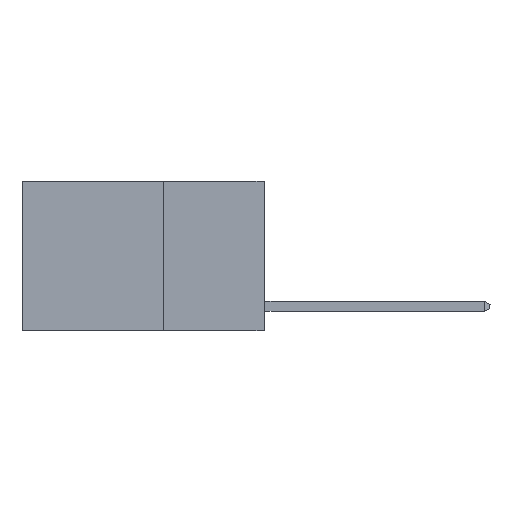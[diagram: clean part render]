
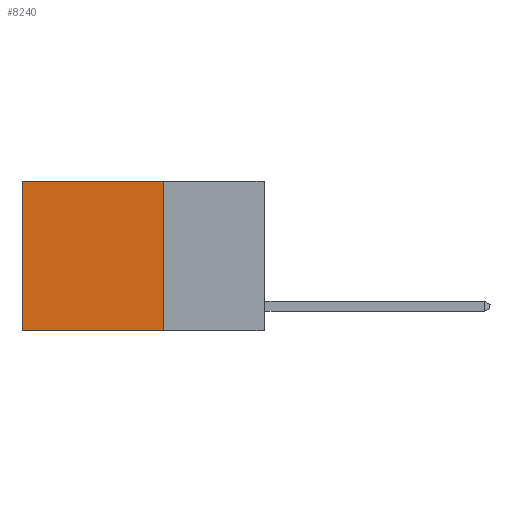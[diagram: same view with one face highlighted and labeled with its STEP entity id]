
A CAD part, left-side view. The second image highlights one B-rep face of the part: STEP entity #8240.
In plain terms, the highlighted planar face has unit normal (-1, 0, 0).
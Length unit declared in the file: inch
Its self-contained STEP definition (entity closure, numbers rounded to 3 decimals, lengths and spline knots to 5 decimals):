
#492 = EDGE_CURVE ( 'NONE', #12961, #1745, #1824, .T. ) ;
#1249 = CARTESIAN_POINT ( 'NONE',  ( 0.2625, 0.6, 0. ) ) ;
#1745 = VERTEX_POINT ( 'NONE', #5249 ) ;
#1824 = LINE ( 'NONE', #2599, #2035 ) ;
#2035 = VECTOR ( 'NONE', #9321, 39.37008 ) ;
#2599 = CARTESIAN_POINT ( 'NONE',  ( 0.2625, 0.25, 0. ) ) ;
#2711 = DIRECTION ( 'NONE',  ( 0., 0., -1. ) ) ;
#3293 = ORIENTED_EDGE ( 'NONE', *, *, #17149, .F. ) ;
#3685 = DIRECTION ( 'NONE',  ( 0., 0., -1. ) ) ;
#4154 = CARTESIAN_POINT ( 'NONE',  ( 0.2625, 0.25, 0. ) ) ;
#4544 = CARTESIAN_POINT ( 'NONE',  ( 0.2625, 0.25, 0. ) ) ;
#4685 = AXIS2_PLACEMENT_3D ( 'NONE', #4154, #12245, #13655 ) ;
#4705 = ORIENTED_EDGE ( 'NONE', *, *, #8080, .F. ) ;
#4832 = CARTESIAN_POINT ( 'NONE',  ( 0.2625, 0.6, -0.37 ) ) ;
#5249 = CARTESIAN_POINT ( 'NONE',  ( 0.2625, 0.6, 0. ) ) ;
#6336 = CARTESIAN_POINT ( 'NONE',  ( 0.2625, 0.25, -0.37 ) ) ;
#6711 = FACE_OUTER_BOUND ( 'NONE', #11072, .T. ) ;
#7465 = LINE ( 'NONE', #1249, #8313 ) ;
#8080 = EDGE_CURVE ( 'NONE', #12961, #11526, #13104, .T. ) ;
#8092 = ORIENTED_EDGE ( 'NONE', *, *, #492, .T. ) ;
#8240 = ADVANCED_FACE ( 'NONE', ( #6711 ), #12298, .F. ) ;
#8313 = VECTOR ( 'NONE', #2711, 39.37008 ) ;
#8532 = LINE ( 'NONE', #11748, #8749 ) ;
#8749 = VECTOR ( 'NONE', #15796, 39.37008 ) ;
#8997 = VERTEX_POINT ( 'NONE', #4832 ) ;
#9321 = DIRECTION ( 'NONE',  ( 0., 1., 0. ) ) ;
#11072 = EDGE_LOOP ( 'NONE', ( #14441, #3293, #4705, #8092 ) ) ;
#11526 = VERTEX_POINT ( 'NONE', #6336 ) ;
#11748 = CARTESIAN_POINT ( 'NONE',  ( 0.2625, 0.25, -0.37 ) ) ;
#12245 = DIRECTION ( 'NONE',  ( 1., 0., 0. ) ) ;
#12298 = PLANE ( 'NONE',  #4685 ) ;
#12882 = VECTOR ( 'NONE', #3685, 39.37008 ) ;
#12961 = VERTEX_POINT ( 'NONE', #4544 ) ;
#13104 = LINE ( 'NONE', #13315, #12882 ) ;
#13315 = CARTESIAN_POINT ( 'NONE',  ( 0.2625, 0.25, 0. ) ) ;
#13655 = DIRECTION ( 'NONE',  ( 0., 0., -1. ) ) ;
#14441 = ORIENTED_EDGE ( 'NONE', *, *, #17495, .T. ) ;
#15796 = DIRECTION ( 'NONE',  ( 0., 1., 0. ) ) ;
#17149 = EDGE_CURVE ( 'NONE', #11526, #8997, #8532, .T. ) ;
#17495 = EDGE_CURVE ( 'NONE', #1745, #8997, #7465, .T. ) ;
